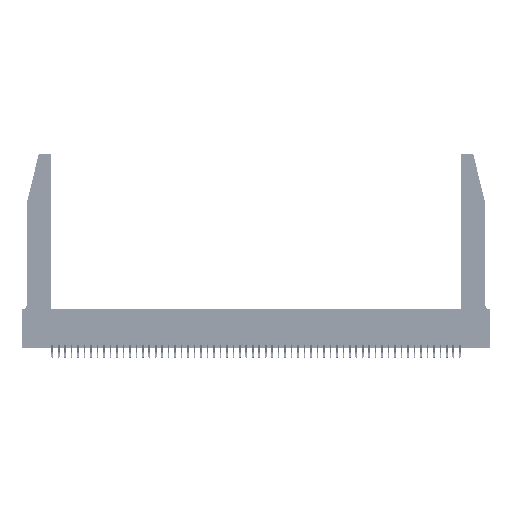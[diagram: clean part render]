
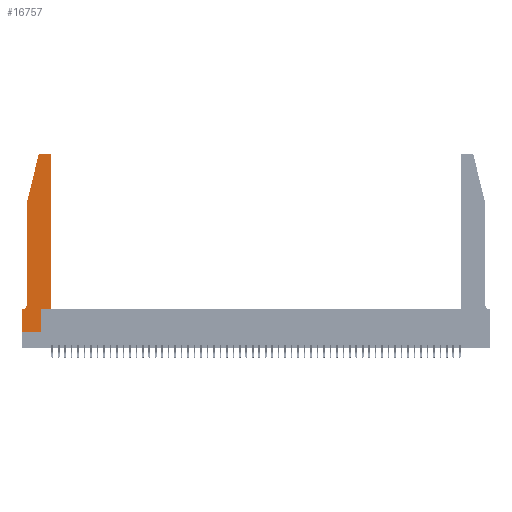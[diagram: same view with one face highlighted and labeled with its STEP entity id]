
A CAD part, top view. The second image highlights one B-rep face of the part: STEP entity #16757.
In plain terms, the highlighted planar face has unit normal (0, 0, 1).
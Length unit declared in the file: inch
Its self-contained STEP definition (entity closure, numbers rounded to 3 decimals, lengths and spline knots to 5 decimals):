
#111 = DIRECTION ( 'NONE',  ( -0.239, -0.971, 0. ) ) ;
#1242 = CARTESIAN_POINT ( 'NONE',  ( 0.0755, 0.35, 0.37 ) ) ;
#1453 = VECTOR ( 'NONE', #16404, 39.37008 ) ;
#1628 = EDGE_CURVE ( 'NONE', #51145, #3494, #7132, .T. ) ;
#2803 = DIRECTION ( 'NONE',  ( 1., 0., 0. ) ) ;
#3494 = VERTEX_POINT ( 'NONE', #13709 ) ;
#3572 = PLANE ( 'NONE',  #34222 ) ;
#3752 = DIRECTION ( 'NONE',  ( 1., 0., 0. ) ) ;
#4608 = CIRCLE ( 'NONE', #27765, 0.03 ) ;
#5011 = CARTESIAN_POINT ( 'NONE',  ( 0.4505, 0.35, 0.37 ) ) ;
#5563 = DIRECTION ( 'NONE',  ( 0., 0., 1. ) ) ;
#5677 = DIRECTION ( 'NONE',  ( 0., 0., 1. ) ) ;
#5745 = ORIENTED_EDGE ( 'NONE', *, *, #41840, .T. ) ;
#7132 = LINE ( 'NONE', #1242, #18548 ) ;
#7391 = LINE ( 'NONE', #10045, #48415 ) ;
#7409 = EDGE_CURVE ( 'NONE', #46643, #33033, #13672, .T. ) ;
#7957 = DIRECTION ( 'NONE',  ( 0., 0., 1. ) ) ;
#8128 = CARTESIAN_POINT ( 'NONE',  ( 0., 0.35, 0.37 ) ) ;
#8554 = EDGE_CURVE ( 'NONE', #33033, #20222, #41877, .T. ) ;
#8889 = ORIENTED_EDGE ( 'NONE', *, *, #8966, .T. ) ;
#8966 = EDGE_CURVE ( 'NONE', #20222, #39433, #4608, .T. ) ;
#9063 = VECTOR ( 'NONE', #49468, 39.37008 ) ;
#9204 = CARTESIAN_POINT ( 'NONE',  ( 0.284, 2.72, 0.37 ) ) ;
#9510 = CARTESIAN_POINT ( 'NONE',  ( 0.0055, 0.42, 0.37 ) ) ;
#9872 = DIRECTION ( 'NONE',  ( 0., -1., 0. ) ) ;
#10045 = CARTESIAN_POINT ( 'NONE',  ( 0.2865, 0.35, 0.37 ) ) ;
#10491 = CARTESIAN_POINT ( 'NONE',  ( 0.4205, 2.75, 0.37 ) ) ;
#11209 = CARTESIAN_POINT ( 'NONE',  ( 0.2865, 0., 0.37 ) ) ;
#11230 = CARTESIAN_POINT ( 'NONE',  ( 0.2605, 2.75, 0.37 ) ) ;
#11272 = LINE ( 'NONE', #36278, #38383 ) ;
#11787 = CARTESIAN_POINT ( 'NONE',  ( 0.0755, 2., 0.37 ) ) ;
#12163 = EDGE_CURVE ( 'NONE', #33104, #51145, #43129, .T. ) ;
#13591 = CARTESIAN_POINT ( 'NONE',  ( 0., 0., 0.37 ) ) ;
#13672 = CIRCLE ( 'NONE', #24368, 0.03 ) ;
#13709 = CARTESIAN_POINT ( 'NONE',  ( 0., 0.35, 0.37 ) ) ;
#14636 = VERTEX_POINT ( 'NONE', #11209 ) ;
#15124 = ORIENTED_EDGE ( 'NONE', *, *, #8554, .T. ) ;
#15264 = DIRECTION ( 'NONE',  ( -1., 0., 0. ) ) ;
#15387 = EDGE_CURVE ( 'NONE', #51600, #33104, #35847, .T. ) ;
#15602 = LINE ( 'NONE', #13591, #49037 ) ;
#15947 = CARTESIAN_POINT ( 'NONE',  ( 0.2865, 0.35, 0.37 ) ) ;
#16404 = DIRECTION ( 'NONE',  ( 1., 0., 0. ) ) ;
#16757 = ADVANCED_FACE ( 'NONE', ( #31266 ), #3572, .T. ) ;
#16913 = VECTOR ( 'NONE', #31571, 39.37008 ) ;
#17801 = CARTESIAN_POINT ( 'NONE',  ( 0.284, 2.75, 0.37 ) ) ;
#17981 = DIRECTION ( 'NONE',  ( 0., 0., -1. ) ) ;
#18548 = VECTOR ( 'NONE', #25915, 39.37008 ) ;
#19807 = ORIENTED_EDGE ( 'NONE', *, *, #47903, .T. ) ;
#19819 = LINE ( 'NONE', #40681, #9063 ) ;
#20222 = VERTEX_POINT ( 'NONE', #17801 ) ;
#20288 = EDGE_CURVE ( 'NONE', #14636, #33340, #7391, .T. ) ;
#21359 = EDGE_CURVE ( 'NONE', #3494, #21588, #15602, .T. ) ;
#21411 = DIRECTION ( 'NONE',  ( 1., 0., 0. ) ) ;
#21471 = DIRECTION ( 'NONE',  ( 1., 0., 0. ) ) ;
#21588 = VERTEX_POINT ( 'NONE', #50808 ) ;
#23143 = ORIENTED_EDGE ( 'NONE', *, *, #12163, .T. ) ;
#23634 = CARTESIAN_POINT ( 'NONE',  ( 0.0755, 2., 0.37 ) ) ;
#24368 = AXIS2_PLACEMENT_3D ( 'NONE', #33967, #5563, #21471 ) ;
#25915 = DIRECTION ( 'NONE',  ( -1., 0., 0. ) ) ;
#26085 = DIRECTION ( 'NONE',  ( 0., 1., 0. ) ) ;
#26989 = ORIENTED_EDGE ( 'NONE', *, *, #21359, .T. ) ;
#27765 = AXIS2_PLACEMENT_3D ( 'NONE', #9204, #5677, #21411 ) ;
#28027 = CARTESIAN_POINT ( 'NONE',  ( 0., 0., 0.37 ) ) ;
#29303 = ORIENTED_EDGE ( 'NONE', *, *, #20288, .T. ) ;
#29660 = ORIENTED_EDGE ( 'NONE', *, *, #1628, .T. ) ;
#30926 = LINE ( 'NONE', #43565, #36600 ) ;
#31123 = LINE ( 'NONE', #28027, #1453 ) ;
#31266 = FACE_OUTER_BOUND ( 'NONE', #42569, .T. ) ;
#31571 = DIRECTION ( 'NONE',  ( 0., -1., 0. ) ) ;
#31850 = ORIENTED_EDGE ( 'NONE', *, *, #39958, .T. ) ;
#33033 = VERTEX_POINT ( 'NONE', #10491 ) ;
#33104 = VERTEX_POINT ( 'NONE', #39561 ) ;
#33340 = VERTEX_POINT ( 'NONE', #15947 ) ;
#33967 = CARTESIAN_POINT ( 'NONE',  ( 0.4205, 2.72, 0.37 ) ) ;
#34222 = AXIS2_PLACEMENT_3D ( 'NONE', #8128, #7957, #3752 ) ;
#34314 = CARTESIAN_POINT ( 'NONE',  ( 0.4505, 2.72, 0.37 ) ) ;
#34705 = ORIENTED_EDGE ( 'NONE', *, *, #15387, .T. ) ;
#35847 = LINE ( 'NONE', #23634, #16913 ) ;
#36278 = CARTESIAN_POINT ( 'NONE',  ( 0.0755, 2., 0.37 ) ) ;
#36370 = CARTESIAN_POINT ( 'NONE',  ( 0.25487, 2.72718, 0.37 ) ) ;
#36600 = VECTOR ( 'NONE', #2803, 39.37008 ) ;
#38277 = DIRECTION ( 'NONE',  ( -1., 0., 0. ) ) ;
#38383 = VECTOR ( 'NONE', #111, 39.37008 ) ;
#39433 = VERTEX_POINT ( 'NONE', #36370 ) ;
#39471 = AXIS2_PLACEMENT_3D ( 'NONE', #9510, #17981, #38277 ) ;
#39561 = CARTESIAN_POINT ( 'NONE',  ( 0.0755, 0.42, 0.37 ) ) ;
#39958 = EDGE_CURVE ( 'NONE', #21588, #14636, #31123, .T. ) ;
#40681 = CARTESIAN_POINT ( 'NONE',  ( 0.4505, 0.35, 0.37 ) ) ;
#41597 = CARTESIAN_POINT ( 'NONE',  ( 0.0055, 0.35, 0.37 ) ) ;
#41840 = EDGE_CURVE ( 'NONE', #33340, #49132, #30926, .T. ) ;
#41877 = LINE ( 'NONE', #11230, #46309 ) ;
#42569 = EDGE_LOOP ( 'NONE', ( #15124, #8889, #42878, #34705, #23143, #29660, #26989, #31850, #29303, #5745, #19807, #47935 ) ) ;
#42688 = EDGE_CURVE ( 'NONE', #39433, #51600, #11272, .T. ) ;
#42878 = ORIENTED_EDGE ( 'NONE', *, *, #42688, .T. ) ;
#43129 = CIRCLE ( 'NONE', #39471, 0.07 ) ;
#43565 = CARTESIAN_POINT ( 'NONE',  ( 0.4505, 0.35, 0.37 ) ) ;
#46309 = VECTOR ( 'NONE', #15264, 39.37008 ) ;
#46643 = VERTEX_POINT ( 'NONE', #34314 ) ;
#47903 = EDGE_CURVE ( 'NONE', #49132, #46643, #19819, .T. ) ;
#47935 = ORIENTED_EDGE ( 'NONE', *, *, #7409, .T. ) ;
#48415 = VECTOR ( 'NONE', #26085, 39.37008 ) ;
#49037 = VECTOR ( 'NONE', #9872, 39.37008 ) ;
#49132 = VERTEX_POINT ( 'NONE', #5011 ) ;
#49468 = DIRECTION ( 'NONE',  ( 0., 1., 0. ) ) ;
#50808 = CARTESIAN_POINT ( 'NONE',  ( 0., 0., 0.37 ) ) ;
#51145 = VERTEX_POINT ( 'NONE', #41597 ) ;
#51600 = VERTEX_POINT ( 'NONE', #11787 ) ;
